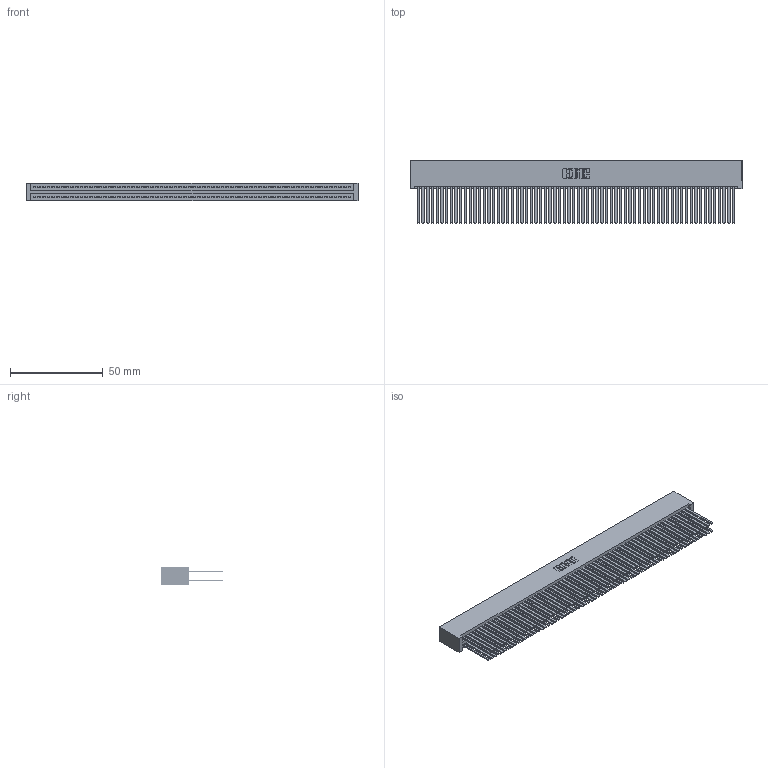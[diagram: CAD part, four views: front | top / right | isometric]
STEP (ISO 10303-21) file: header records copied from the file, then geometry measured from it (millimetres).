
FILE_DESCRIPTION (( 'STEP AP203' ), '1' );
FILE_NAME ('345-136-544-201.STEP', '2018-10-20T14:36:18', ( '' ), ( '' ), 'SwSTEP 2.0', 'SolidWorks 2016', '' );
FILE_SCHEMA (( 'CONFIG_CONTROL_DESIGN' ));
Length unit declared in the file: inch
Products named in the file (3): 345 Part_No Mounting Lugs; 345-136-544-201; 345-292-001_345-293-144
Assembly tree (137 placements, depth 2):
  345-136-544-201
    345 Part_No Mounting Lugs
    345-292-001_345-293-144  x136
Bounding box: 179.32 x 33.96 x 9.4 mm (x, y, z)
Volume: 20183.4 mm3; surface area: 36229 mm2
Topology: 137 solids, 137 shells, 6102 faces, 18133 edges, 11906 vertices
Faces by surface type: plane 4020, cylinder 2082
Entity records: 49393 total; most frequent: CARTESIAN_POINT 8252, ORIENTED_EDGE 8186, DIRECTION 7237, EDGE_CURVE 4093, VECTOR 3701, LINE 3701, VERTEX_POINT 2726, AXIS2_PLACEMENT_3D 1768
